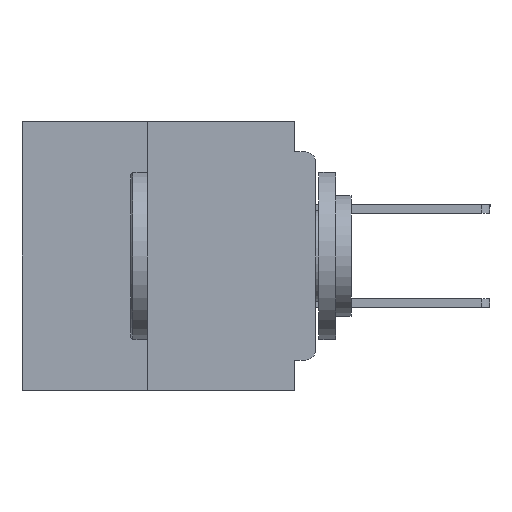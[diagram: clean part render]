
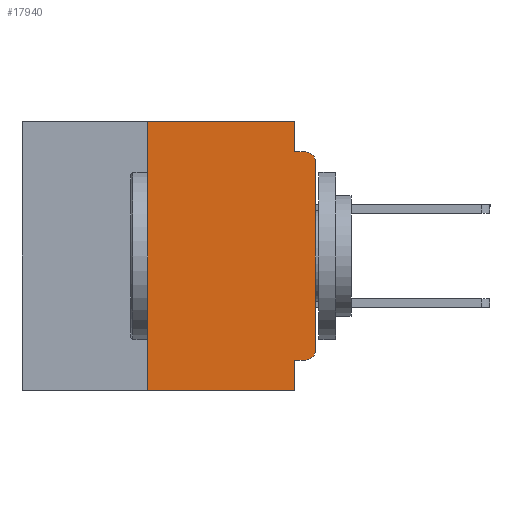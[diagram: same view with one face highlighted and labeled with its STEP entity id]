
A CAD part, left-side view. The second image highlights one B-rep face of the part: STEP entity #17940.
In plain terms, the highlighted planar face has unit normal (-1, 0, 0).
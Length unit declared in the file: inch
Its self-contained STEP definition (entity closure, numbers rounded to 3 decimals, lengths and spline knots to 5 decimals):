
#9 = ORIENTED_EDGE ( 'NONE', *, *, #44061, .F. ) ;
#1622 = LINE ( 'NONE', #56372, #3253 ) ;
#2086 = CARTESIAN_POINT ( 'NONE',  ( 0., 0.031, 0. ) ) ;
#3253 = VECTOR ( 'NONE', #35844, 39.37008 ) ;
#3930 = DIRECTION ( 'NONE',  ( -1., 0., 0. ) ) ;
#3937 = LINE ( 'NONE', #52020, #28245 ) ;
#4953 = CARTESIAN_POINT ( 'NONE',  ( 0., 0.031, 0. ) ) ;
#5546 = DIRECTION ( 'NONE',  ( -1., 0., 0. ) ) ;
#5679 = DIRECTION ( 'NONE',  ( 0., 0., 1. ) ) ;
#7542 = CARTESIAN_POINT ( 'NONE',  ( 0., 0.015, -0.045 ) ) ;
#8715 = EDGE_CURVE ( 'NONE', #18949, #28649, #64332, .T. ) ;
#9030 = CARTESIAN_POINT ( 'NONE',  ( 0., 0., -0.06 ) ) ;
#9255 = CARTESIAN_POINT ( 'NONE',  ( 0., 0.437, -0.4 ) ) ;
#10161 = VERTEX_POINT ( 'NONE', #29631 ) ;
#11176 = VERTEX_POINT ( 'NONE', #12075 ) ;
#12075 = CARTESIAN_POINT ( 'NONE',  ( 0., 0.031, -0.355 ) ) ;
#12654 = VECTOR ( 'NONE', #36883, 39.37008 ) ;
#12787 = CARTESIAN_POINT ( 'NONE',  ( 0., 0.437, 0. ) ) ;
#13574 = ORIENTED_EDGE ( 'NONE', *, *, #18957, .T. ) ;
#13784 = CARTESIAN_POINT ( 'NONE',  ( 0., 0., -0.355 ) ) ;
#14757 = EDGE_CURVE ( 'NONE', #52834, #20263, #29231, .T. ) ;
#15936 = AXIS2_PLACEMENT_3D ( 'NONE', #34934, #3930, #40065 ) ;
#16029 = CARTESIAN_POINT ( 'NONE',  ( 0., 0.015, -0.355 ) ) ;
#16565 = LINE ( 'NONE', #12787, #54516 ) ;
#16659 = PLANE ( 'NONE',  #66077 ) ;
#16924 = EDGE_CURVE ( 'NONE', #10161, #28649, #48463, .T. ) ;
#17940 = ADVANCED_FACE ( 'NONE', ( #53914 ), #16659, .F. ) ;
#18910 = ORIENTED_EDGE ( 'NONE', *, *, #14757, .T. ) ;
#18949 = VERTEX_POINT ( 'NONE', #9030 ) ;
#18957 = EDGE_CURVE ( 'NONE', #33375, #60898, #22638, .T. ) ;
#20099 = LINE ( 'NONE', #13784, #32202 ) ;
#20263 = VERTEX_POINT ( 'NONE', #29479 ) ;
#20453 = EDGE_CURVE ( 'NONE', #11176, #60898, #40110, .T. ) ;
#21871 = DIRECTION ( 'NONE',  ( 0., 0., -1. ) ) ;
#22638 = LINE ( 'NONE', #9255, #34733 ) ;
#24465 = VECTOR ( 'NONE', #48685, 39.37008 ) ;
#26407 = ORIENTED_EDGE ( 'NONE', *, *, #8715, .T. ) ;
#27203 = ORIENTED_EDGE ( 'NONE', *, *, #27528, .F. ) ;
#27528 = EDGE_CURVE ( 'NONE', #52834, #11176, #20099, .T. ) ;
#28163 = EDGE_LOOP ( 'NONE', ( #48555, #26407, #65598, #9, #61494, #40620, #13574, #35344, #27203, #18910 ) ) ;
#28245 = VECTOR ( 'NONE', #5679, 39.37008 ) ;
#28649 = VERTEX_POINT ( 'NONE', #7542 ) ;
#29231 = CIRCLE ( 'NONE', #49111, 0.015 ) ;
#29479 = CARTESIAN_POINT ( 'NONE',  ( 0., 0., -0.34 ) ) ;
#29631 = CARTESIAN_POINT ( 'NONE',  ( 0., 0.031, -0.045 ) ) ;
#30134 = DIRECTION ( 'NONE',  ( 0., -1., 0. ) ) ;
#31705 = CARTESIAN_POINT ( 'NONE',  ( 0., 0.031, -0.4 ) ) ;
#32202 = VECTOR ( 'NONE', #54902, 39.37008 ) ;
#32428 = EDGE_CURVE ( 'NONE', #44277, #59444, #16565, .T. ) ;
#33375 = VERTEX_POINT ( 'NONE', #45669 ) ;
#34733 = VECTOR ( 'NONE', #45425, 39.37008 ) ;
#34934 = CARTESIAN_POINT ( 'NONE',  ( 0., 0.015, -0.06 ) ) ;
#35344 = ORIENTED_EDGE ( 'NONE', *, *, #20453, .F. ) ;
#35844 = DIRECTION ( 'NONE',  ( 0., 0., 1. ) ) ;
#36517 = CARTESIAN_POINT ( 'NONE',  ( 0., 0.015, -0.34 ) ) ;
#36883 = DIRECTION ( 'NONE',  ( 0., 0., -1. ) ) ;
#38612 = EDGE_CURVE ( 'NONE', #20263, #18949, #3937, .T. ) ;
#38748 = DIRECTION ( 'NONE',  ( 0., -1., 0. ) ) ;
#40065 = DIRECTION ( 'NONE',  ( 0., 0., -1. ) ) ;
#40110 = LINE ( 'NONE', #31705, #12654 ) ;
#40620 = ORIENTED_EDGE ( 'NONE', *, *, #52463, .F. ) ;
#41702 = DIRECTION ( 'NONE',  ( 0., 0., -1. ) ) ;
#42371 = CARTESIAN_POINT ( 'NONE',  ( 0., 0.437, 0. ) ) ;
#44061 = EDGE_CURVE ( 'NONE', #59444, #10161, #51905, .T. ) ;
#44277 = VERTEX_POINT ( 'NONE', #48035 ) ;
#45425 = DIRECTION ( 'NONE',  ( 0., -1., 0. ) ) ;
#45669 = CARTESIAN_POINT ( 'NONE',  ( 0., 0.25, -0.4 ) ) ;
#48035 = CARTESIAN_POINT ( 'NONE',  ( 0., 0.25, 0. ) ) ;
#48463 = LINE ( 'NONE', #55843, #58899 ) ;
#48555 = ORIENTED_EDGE ( 'NONE', *, *, #38612, .T. ) ;
#48685 = DIRECTION ( 'NONE',  ( 0., 0., -1. ) ) ;
#49111 = AXIS2_PLACEMENT_3D ( 'NONE', #36517, #5546, #41702 ) ;
#51905 = LINE ( 'NONE', #2086, #24465 ) ;
#52020 = CARTESIAN_POINT ( 'NONE',  ( 0., 0., 0. ) ) ;
#52463 = EDGE_CURVE ( 'NONE', #33375, #44277, #1622, .T. ) ;
#52765 = DIRECTION ( 'NONE',  ( 1., 0., 0. ) ) ;
#52834 = VERTEX_POINT ( 'NONE', #16029 ) ;
#53914 = FACE_OUTER_BOUND ( 'NONE', #28163, .T. ) ;
#54516 = VECTOR ( 'NONE', #38748, 39.37008 ) ;
#54902 = DIRECTION ( 'NONE',  ( 0., 1., 0. ) ) ;
#55843 = CARTESIAN_POINT ( 'NONE',  ( 0., 0., -0.045 ) ) ;
#56372 = CARTESIAN_POINT ( 'NONE',  ( 0., 0.25, -0.4 ) ) ;
#58899 = VECTOR ( 'NONE', #30134, 39.37008 ) ;
#59444 = VERTEX_POINT ( 'NONE', #4953 ) ;
#60898 = VERTEX_POINT ( 'NONE', #63079 ) ;
#61494 = ORIENTED_EDGE ( 'NONE', *, *, #32428, .F. ) ;
#63079 = CARTESIAN_POINT ( 'NONE',  ( 0., 0.031, -0.4 ) ) ;
#64332 = CIRCLE ( 'NONE', #15936, 0.015 ) ;
#65598 = ORIENTED_EDGE ( 'NONE', *, *, #16924, .F. ) ;
#66077 = AXIS2_PLACEMENT_3D ( 'NONE', #42371, #52765, #21871 ) ;
